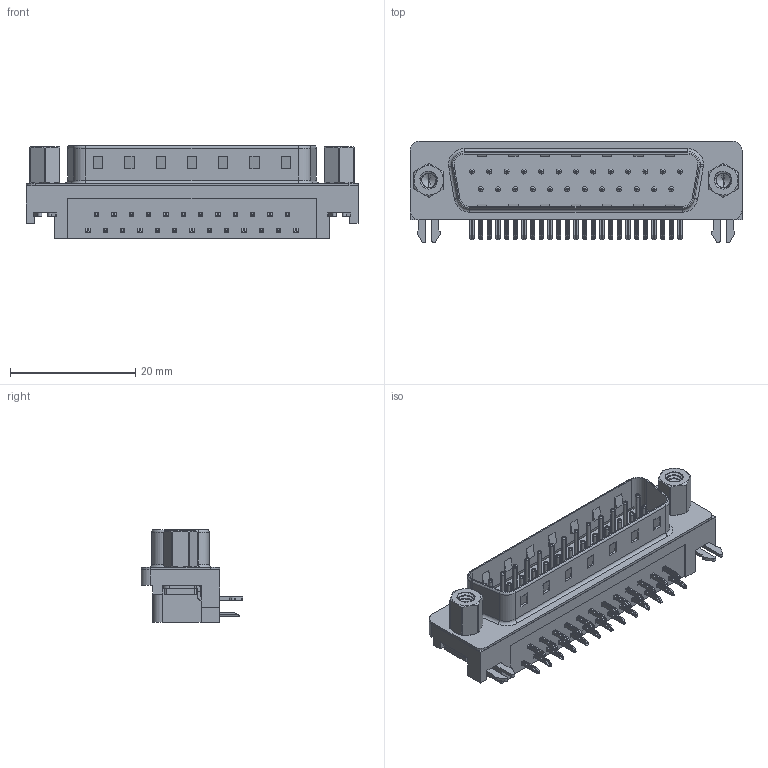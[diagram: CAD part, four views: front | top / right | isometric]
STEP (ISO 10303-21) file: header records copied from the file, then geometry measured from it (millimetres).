
FILE_DESCRIPTION (( 'STEP AP203' ), '1' );
FILE_NAME ('623-025-661-533.STEP', '2018-11-06T13:08:07', ( '' ), ( '' ), 'SwSTEP 2.0', 'SolidWorks 2016', '' );
FILE_SCHEMA (( 'CONFIG_CONTROL_DESIGN' ));
Length unit declared in the file: millimetre
Products named in the file (8): 623 Contact Bottom; 623 Contact Top; 623 2 Prong Board Lock; 623 4-40 Threaded Rivet; 623 4-40 Hex Standoff 5; 623-025-661-533; 623 Housing_25 Socket; 623 Shell_25 Socket
Assembly tree (33 placements, depth 2):
  623-025-661-533
    623 Housing_25 Socket
    623 Shell_25 Socket
    623 Contact Bottom  x12
    623 Contact Top  x13
    623 2 Prong Board Lock  x2
    623 4-40 Threaded Rivet  x2
    623 4-40 Hex Standoff 5  x2
Bounding box: 53.04 x 16.25 x 14.8 mm (x, y, z)
Volume: 4942.2 mm3; surface area: 7249.2 mm2
Topology: 33 solids, 33 shells, 2409 faces, 6003 edges, 3721 vertices
Faces by surface type: plane 1455, cylinder 721, torus 181, cone 34, bspline 18
Entity records: 27426 total; most frequent: CARTESIAN_POINT 8362, DIRECTION 3634, ORIENTED_EDGE 3624, EDGE_CURVE 1812, VECTOR 1224, LINE 1224, AXIS2_PLACEMENT_3D 1205, VERTEX_POINT 1165
